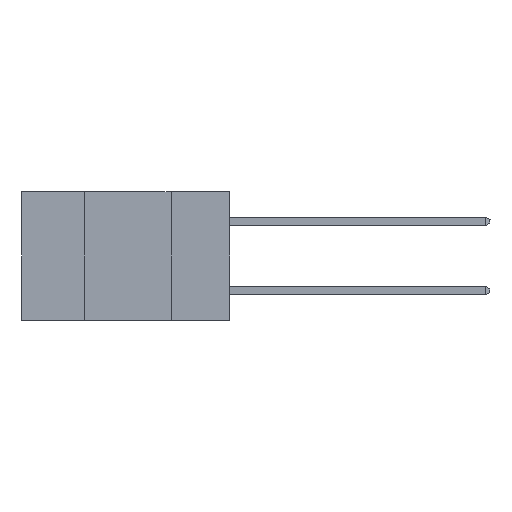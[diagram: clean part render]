
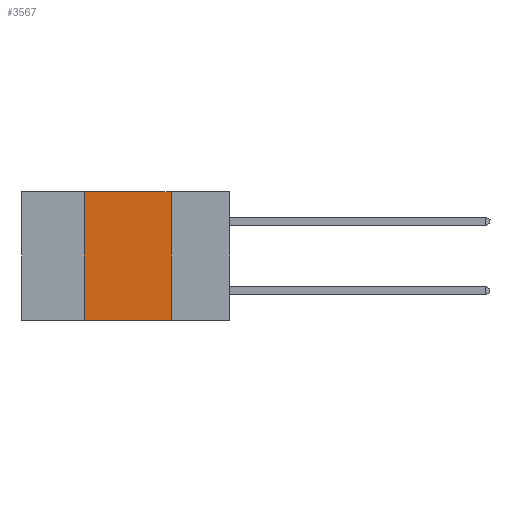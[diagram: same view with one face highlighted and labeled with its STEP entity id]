
A CAD part, left-side view. The second image highlights one B-rep face of the part: STEP entity #3567.
In plain terms, the highlighted planar face has unit normal (-1, 0, 0).
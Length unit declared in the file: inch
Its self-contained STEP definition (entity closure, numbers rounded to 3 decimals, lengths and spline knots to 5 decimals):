
#547 = CARTESIAN_POINT ( 'NONE',  ( 0., 0.17, 0. ) ) ;
#808 = ORIENTED_EDGE ( 'NONE', *, *, #10245, .F. ) ;
#859 = VERTEX_POINT ( 'NONE', #14022 ) ;
#872 = LINE ( 'NONE', #6795, #7314 ) ;
#1334 = CARTESIAN_POINT ( 'NONE',  ( 0., 0.17, -0.37 ) ) ;
#1582 = DIRECTION ( 'NONE',  ( 0., 0., 1. ) ) ;
#1768 = VERTEX_POINT ( 'NONE', #7615 ) ;
#2469 = CARTESIAN_POINT ( 'NONE',  ( 0., 0.6, -0.37 ) ) ;
#3030 = LINE ( 'NONE', #2469, #4871 ) ;
#3174 = DIRECTION ( 'NONE',  ( 0., 0., -1. ) ) ;
#3567 = ADVANCED_FACE ( 'NONE', ( #7961 ), #8314, .F. ) ;
#3852 = CARTESIAN_POINT ( 'NONE',  ( 0., 0.6, 0. ) ) ;
#4871 = VECTOR ( 'NONE', #11744, 39.37008 ) ;
#5112 = EDGE_CURVE ( 'NONE', #9726, #14139, #8342, .T. ) ;
#6795 = CARTESIAN_POINT ( 'NONE',  ( 0., 0.42, 0. ) ) ;
#7314 = VECTOR ( 'NONE', #1582, 39.37008 ) ;
#7615 = CARTESIAN_POINT ( 'NONE',  ( 0., 0.42, 0. ) ) ;
#7961 = FACE_OUTER_BOUND ( 'NONE', #10478, .T. ) ;
#8261 = DIRECTION ( 'NONE',  ( 0., 0., -1. ) ) ;
#8314 = PLANE ( 'NONE',  #9403 ) ;
#8342 = LINE ( 'NONE', #8490, #11874 ) ;
#8490 = CARTESIAN_POINT ( 'NONE',  ( 0., 0.17, 0. ) ) ;
#9403 = AXIS2_PLACEMENT_3D ( 'NONE', #9892, #16753, #3174 ) ;
#9607 = EDGE_CURVE ( 'NONE', #859, #14139, #3030, .T. ) ;
#9726 = VERTEX_POINT ( 'NONE', #547 ) ;
#9806 = ORIENTED_EDGE ( 'NONE', *, *, #5112, .F. ) ;
#9892 = CARTESIAN_POINT ( 'NONE',  ( 0., 0.6, 0. ) ) ;
#10245 = EDGE_CURVE ( 'NONE', #1768, #9726, #11091, .T. ) ;
#10247 = VECTOR ( 'NONE', #15770, 39.37008 ) ;
#10478 = EDGE_LOOP ( 'NONE', ( #9806, #808, #11518, #16216 ) ) ;
#10980 = EDGE_CURVE ( 'NONE', #859, #1768, #872, .T. ) ;
#11091 = LINE ( 'NONE', #3852, #10247 ) ;
#11518 = ORIENTED_EDGE ( 'NONE', *, *, #10980, .F. ) ;
#11744 = DIRECTION ( 'NONE',  ( 0., -1., 0. ) ) ;
#11874 = VECTOR ( 'NONE', #8261, 39.37008 ) ;
#14022 = CARTESIAN_POINT ( 'NONE',  ( 0., 0.42, -0.37 ) ) ;
#14139 = VERTEX_POINT ( 'NONE', #1334 ) ;
#15770 = DIRECTION ( 'NONE',  ( 0., -1., 0. ) ) ;
#16216 = ORIENTED_EDGE ( 'NONE', *, *, #9607, .T. ) ;
#16753 = DIRECTION ( 'NONE',  ( 1., 0., 0. ) ) ;
